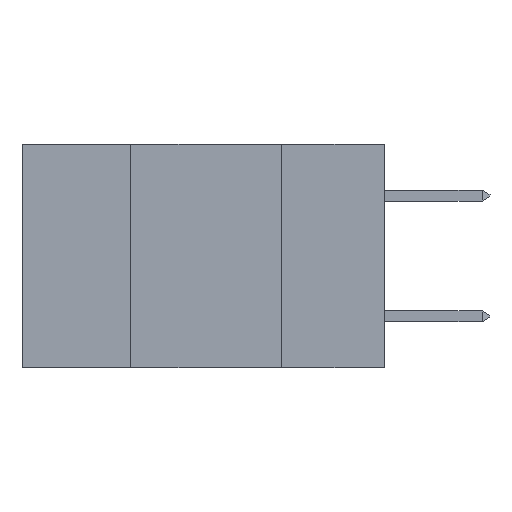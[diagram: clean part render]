
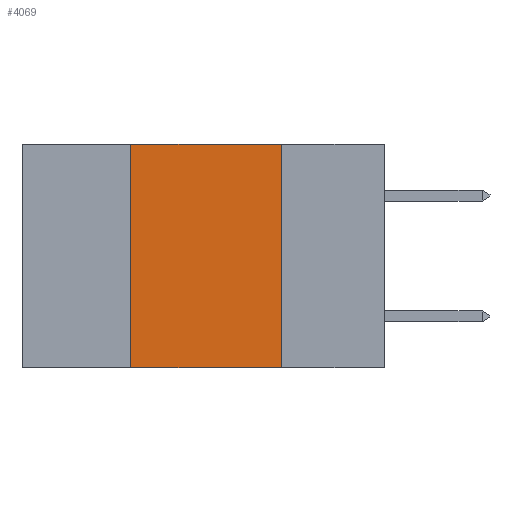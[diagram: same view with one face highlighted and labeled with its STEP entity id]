
A CAD part, left-side view. The second image highlights one B-rep face of the part: STEP entity #4069.
In plain terms, the highlighted planar face has unit normal (-1, 0, 0).
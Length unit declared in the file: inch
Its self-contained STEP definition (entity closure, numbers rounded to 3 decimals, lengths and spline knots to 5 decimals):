
#159 = VERTEX_POINT ( 'NONE', #17791 ) ;
#303 = PLANE ( 'NONE',  #19773 ) ;
#430 = EDGE_CURVE ( 'NONE', #159, #17326, #7658, .T. ) ;
#1188 = VERTEX_POINT ( 'NONE', #15132 ) ;
#2036 = DIRECTION ( 'NONE',  ( 0., 0., -1. ) ) ;
#2145 = CARTESIAN_POINT ( 'NONE',  ( 0., 0.17, -0.37 ) ) ;
#3256 = EDGE_CURVE ( 'NONE', #1188, #12082, #22929, .T. ) ;
#3655 = DIRECTION ( 'NONE',  ( 0., 0., 1. ) ) ;
#4005 = CARTESIAN_POINT ( 'NONE',  ( 0., 0.6, -0.37 ) ) ;
#4069 = ADVANCED_FACE ( 'NONE', ( #10503 ), #303, .F. ) ;
#6005 = DIRECTION ( 'NONE',  ( 0., 0., -1. ) ) ;
#7143 = EDGE_CURVE ( 'NONE', #12082, #17326, #17931, .T. ) ;
#7461 = VECTOR ( 'NONE', #6005, 39.37008 ) ;
#7642 = CARTESIAN_POINT ( 'NONE',  ( 0., 0.6, 0. ) ) ;
#7658 = LINE ( 'NONE', #4005, #11902 ) ;
#7951 = CARTESIAN_POINT ( 'NONE',  ( 0., 0.17, 0. ) ) ;
#8735 = ORIENTED_EDGE ( 'NONE', *, *, #430, .T. ) ;
#8959 = LINE ( 'NONE', #16341, #22775 ) ;
#9712 = CARTESIAN_POINT ( 'NONE',  ( 0., 0.6, 0. ) ) ;
#10503 = FACE_OUTER_BOUND ( 'NONE', #11557, .T. ) ;
#11557 = EDGE_LOOP ( 'NONE', ( #18121, #21358, #16239, #8735 ) ) ;
#11666 = VECTOR ( 'NONE', #13488, 39.37008 ) ;
#11902 = VECTOR ( 'NONE', #21580, 39.37008 ) ;
#12082 = VERTEX_POINT ( 'NONE', #20028 ) ;
#13488 = DIRECTION ( 'NONE',  ( 0., -1., 0. ) ) ;
#15132 = CARTESIAN_POINT ( 'NONE',  ( 0., 0.42, 0. ) ) ;
#15376 = EDGE_CURVE ( 'NONE', #159, #1188, #8959, .T. ) ;
#16239 = ORIENTED_EDGE ( 'NONE', *, *, #15376, .F. ) ;
#16341 = CARTESIAN_POINT ( 'NONE',  ( 0., 0.42, 0. ) ) ;
#16644 = DIRECTION ( 'NONE',  ( 1., 0., 0. ) ) ;
#17326 = VERTEX_POINT ( 'NONE', #2145 ) ;
#17791 = CARTESIAN_POINT ( 'NONE',  ( 0., 0.42, -0.37 ) ) ;
#17931 = LINE ( 'NONE', #7951, #7461 ) ;
#18121 = ORIENTED_EDGE ( 'NONE', *, *, #7143, .F. ) ;
#19773 = AXIS2_PLACEMENT_3D ( 'NONE', #7642, #16644, #2036 ) ;
#20028 = CARTESIAN_POINT ( 'NONE',  ( 0., 0.17, 0. ) ) ;
#21358 = ORIENTED_EDGE ( 'NONE', *, *, #3256, .F. ) ;
#21580 = DIRECTION ( 'NONE',  ( 0., -1., 0. ) ) ;
#22775 = VECTOR ( 'NONE', #3655, 39.37008 ) ;
#22929 = LINE ( 'NONE', #9712, #11666 ) ;
